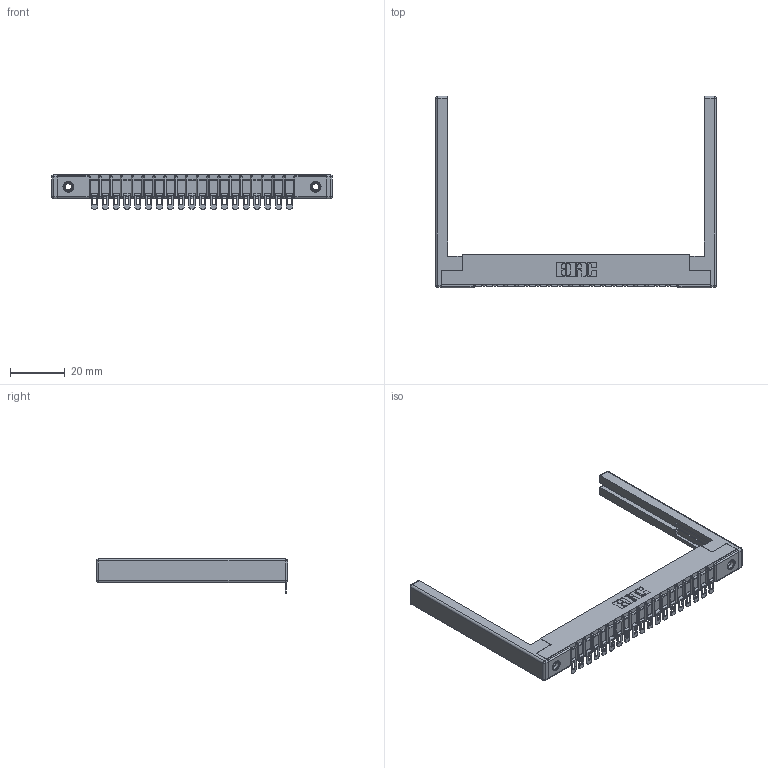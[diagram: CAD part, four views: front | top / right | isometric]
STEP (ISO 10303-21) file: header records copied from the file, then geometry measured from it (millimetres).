
FILE_DESCRIPTION (( 'STEP AP203' ), '1' );
FILE_NAME ('357-019-454-168.STEP', '2020-10-01T02:50:44', ( '' ), ( '' ), 'SwSTEP 2.0', 'SolidWorks 2020', '' );
FILE_SCHEMA (( 'CONFIG_CONTROL_DESIGN' ));
Length unit declared in the file: inch
Products named in the file (5): 307 Part_.156 Dia Mounting Holes; 345-250-001_345-250-001-102; 307-290-002_554; 357-019-454-168; 307-220-068
Assembly tree (24 placements, depth 2):
  357-019-454-168
    307 Part_.156 Dia Mounting Holes
    307-290-002_554  x19
    307-220-068  x2
    345-250-001_345-250-001-102  x2
Bounding box: 102.72 x 69.98 x 12.52 mm (x, y, z)
Volume: 11345.3 mm3; surface area: 16275.4 mm2
Topology: 24 solids, 24 shells, 1831 faces, 5520 edges, 3604 vertices
Faces by surface type: plane 1032, cylinder 735, sphere 48, cone 12, torus 4
Entity records: 22848 total; most frequent: CARTESIAN_POINT 3815, ORIENTED_EDGE 3794, DIRECTION 3741, EDGE_CURVE 1897, LINE 1433, VECTOR 1433, VERTEX_POINT 1228, AXIS2_PLACEMENT_3D 1154
